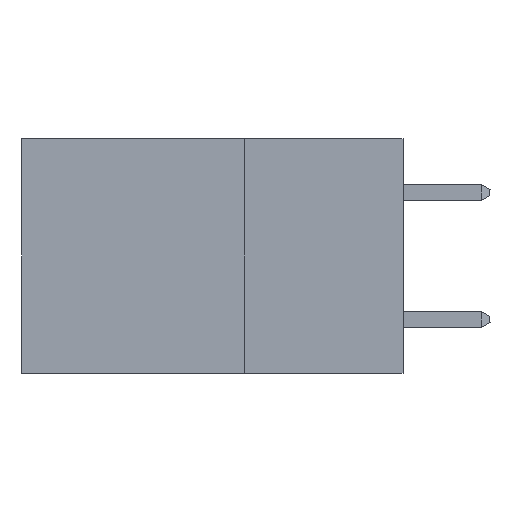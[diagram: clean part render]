
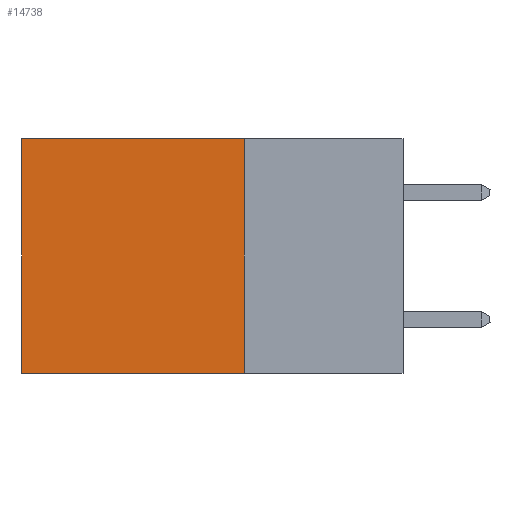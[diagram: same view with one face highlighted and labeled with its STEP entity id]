
A CAD part, left-side view. The second image highlights one B-rep face of the part: STEP entity #14738.
In plain terms, the highlighted planar face has unit normal (-1, 0, 0).
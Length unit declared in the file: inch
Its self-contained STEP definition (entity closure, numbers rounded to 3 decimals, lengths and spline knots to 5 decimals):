
#84 = VERTEX_POINT ( 'NONE', #17638 ) ;
#545 = VECTOR ( 'NONE', #9328, 39.37008 ) ;
#753 = VERTEX_POINT ( 'NONE', #9900 ) ;
#773 = DIRECTION ( 'NONE',  ( 0., 0., -1. ) ) ;
#1203 = ORIENTED_EDGE ( 'NONE', *, *, #18191, .F. ) ;
#1340 = EDGE_CURVE ( 'NONE', #84, #753, #25813, .T. ) ;
#2787 = PLANE ( 'NONE',  #9569 ) ;
#2932 = VECTOR ( 'NONE', #7430, 39.37008 ) ;
#3287 = CARTESIAN_POINT ( 'NONE',  ( 0.2875, 0.6, 0. ) ) ;
#3349 = EDGE_CURVE ( 'NONE', #19135, #14830, #26354, .T. ) ;
#4856 = CARTESIAN_POINT ( 'NONE',  ( 0.2875, 0.25, 0. ) ) ;
#5864 = CARTESIAN_POINT ( 'NONE',  ( 0.2875, 0.25, 0. ) ) ;
#6299 = EDGE_CURVE ( 'NONE', #14830, #753, #13809, .T. ) ;
#7202 = DIRECTION ( 'NONE',  ( 0., 0., -1. ) ) ;
#7430 = DIRECTION ( 'NONE',  ( 0., 1., 0. ) ) ;
#9328 = DIRECTION ( 'NONE',  ( 0., 0., -1. ) ) ;
#9569 = AXIS2_PLACEMENT_3D ( 'NONE', #4856, #13365, #773 ) ;
#9900 = CARTESIAN_POINT ( 'NONE',  ( 0.2875, 0.6, -0.37 ) ) ;
#11192 = CARTESIAN_POINT ( 'NONE',  ( 0.2875, 0.25, 0. ) ) ;
#11214 = VECTOR ( 'NONE', #7202, 39.37008 ) ;
#11521 = ORIENTED_EDGE ( 'NONE', *, *, #6299, .T. ) ;
#13365 = DIRECTION ( 'NONE',  ( 1., 0., 0. ) ) ;
#13809 = LINE ( 'NONE', #3287, #11214 ) ;
#14644 = VECTOR ( 'NONE', #25617, 39.37008 ) ;
#14738 = ADVANCED_FACE ( 'NONE', ( #22324 ), #2787, .F. ) ;
#14830 = VERTEX_POINT ( 'NONE', #22237 ) ;
#16321 = ORIENTED_EDGE ( 'NONE', *, *, #1340, .F. ) ;
#17638 = CARTESIAN_POINT ( 'NONE',  ( 0.2875, 0.25, -0.37 ) ) ;
#17799 = CARTESIAN_POINT ( 'NONE',  ( 0.2875, 0.25, 0. ) ) ;
#18191 = EDGE_CURVE ( 'NONE', #19135, #84, #22805, .T. ) ;
#19135 = VERTEX_POINT ( 'NONE', #11192 ) ;
#20108 = CARTESIAN_POINT ( 'NONE',  ( 0.2875, 0.25, -0.37 ) ) ;
#20949 = EDGE_LOOP ( 'NONE', ( #11521, #16321, #1203, #21536 ) ) ;
#21536 = ORIENTED_EDGE ( 'NONE', *, *, #3349, .T. ) ;
#22237 = CARTESIAN_POINT ( 'NONE',  ( 0.2875, 0.6, 0. ) ) ;
#22324 = FACE_OUTER_BOUND ( 'NONE', #20949, .T. ) ;
#22805 = LINE ( 'NONE', #17799, #545 ) ;
#25617 = DIRECTION ( 'NONE',  ( 0., 1., 0. ) ) ;
#25813 = LINE ( 'NONE', #20108, #2932 ) ;
#26354 = LINE ( 'NONE', #5864, #14644 ) ;
